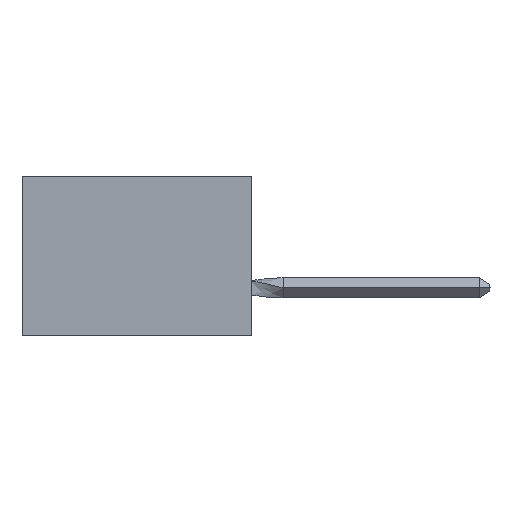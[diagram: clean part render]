
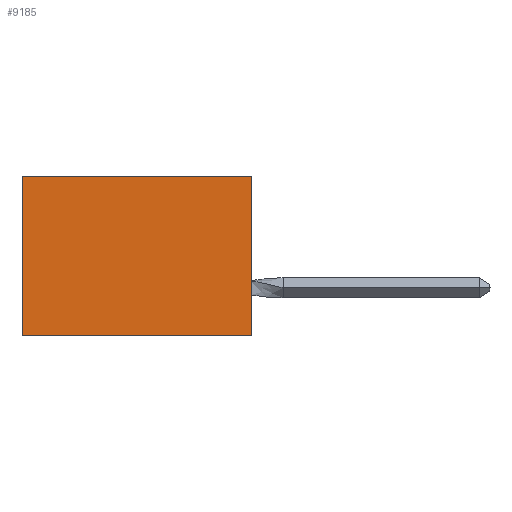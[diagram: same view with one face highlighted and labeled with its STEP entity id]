
A CAD part, left-side view. The second image highlights one B-rep face of the part: STEP entity #9185.
In plain terms, the highlighted planar face has unit normal (-1, 0, 0).
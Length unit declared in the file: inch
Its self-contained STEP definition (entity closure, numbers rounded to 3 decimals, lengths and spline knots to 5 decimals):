
#30 = EDGE_CURVE ( 'NONE', #4403, #6528, #6692, .T. ) ;
#523 = DIRECTION ( 'NONE',  ( 0., 0., -1. ) ) ;
#560 = CARTESIAN_POINT ( 'NONE',  ( 0.305, 0., -0.5 ) ) ;
#1748 = ORIENTED_EDGE ( 'NONE', *, *, #30, .T. ) ;
#1818 = ORIENTED_EDGE ( 'NONE', *, *, #7855, .F. ) ;
#1882 = DIRECTION ( 'NONE',  ( 0., 1., 0. ) ) ;
#2670 = CARTESIAN_POINT ( 'NONE',  ( 0.305, 0., 0. ) ) ;
#3800 = ORIENTED_EDGE ( 'NONE', *, *, #5393, .T. ) ;
#3829 = CARTESIAN_POINT ( 'NONE',  ( 0.305, 0., 0. ) ) ;
#3837 = DIRECTION ( 'NONE',  ( 0., 0., -1. ) ) ;
#3882 = DIRECTION ( 'NONE',  ( 0., 0., -1. ) ) ;
#4403 = VERTEX_POINT ( 'NONE', #3829 ) ;
#4557 = VECTOR ( 'NONE', #4863, 39.37008 ) ;
#4752 = CARTESIAN_POINT ( 'NONE',  ( 0.305, 0.72, -0.5 ) ) ;
#4863 = DIRECTION ( 'NONE',  ( 0., 1., 0. ) ) ;
#5115 = ORIENTED_EDGE ( 'NONE', *, *, #8647, .F. ) ;
#5282 = LINE ( 'NONE', #9871, #10123 ) ;
#5393 = EDGE_CURVE ( 'NONE', #6528, #6828, #11588, .T. ) ;
#5745 = EDGE_LOOP ( 'NONE', ( #3800, #1818, #5115, #1748 ) ) ;
#5789 = PLANE ( 'NONE',  #10563 ) ;
#6391 = VECTOR ( 'NONE', #1882, 39.37008 ) ;
#6528 = VERTEX_POINT ( 'NONE', #12125 ) ;
#6619 = LINE ( 'NONE', #6711, #4557 ) ;
#6692 = LINE ( 'NONE', #2670, #6391 ) ;
#6711 = CARTESIAN_POINT ( 'NONE',  ( 0.305, 0., -0.5 ) ) ;
#6828 = VERTEX_POINT ( 'NONE', #10707 ) ;
#7855 = EDGE_CURVE ( 'NONE', #11144, #6828, #6619, .T. ) ;
#8647 = EDGE_CURVE ( 'NONE', #4403, #11144, #5282, .T. ) ;
#9185 = ADVANCED_FACE ( 'NONE', ( #11145 ), #5789, .F. ) ;
#9521 = DIRECTION ( 'NONE',  ( 1., 0., 0. ) ) ;
#9686 = CARTESIAN_POINT ( 'NONE',  ( 0.305, 0., -0.5 ) ) ;
#9871 = CARTESIAN_POINT ( 'NONE',  ( 0.305, 0., -0.5 ) ) ;
#10123 = VECTOR ( 'NONE', #523, 39.37008 ) ;
#10563 = AXIS2_PLACEMENT_3D ( 'NONE', #9686, #9521, #3882 ) ;
#10570 = VECTOR ( 'NONE', #3837, 39.37008 ) ;
#10707 = CARTESIAN_POINT ( 'NONE',  ( 0.305, 0.72, -0.5 ) ) ;
#11144 = VERTEX_POINT ( 'NONE', #560 ) ;
#11145 = FACE_OUTER_BOUND ( 'NONE', #5745, .T. ) ;
#11588 = LINE ( 'NONE', #4752, #10570 ) ;
#12125 = CARTESIAN_POINT ( 'NONE',  ( 0.305, 0.72, 0. ) ) ;
